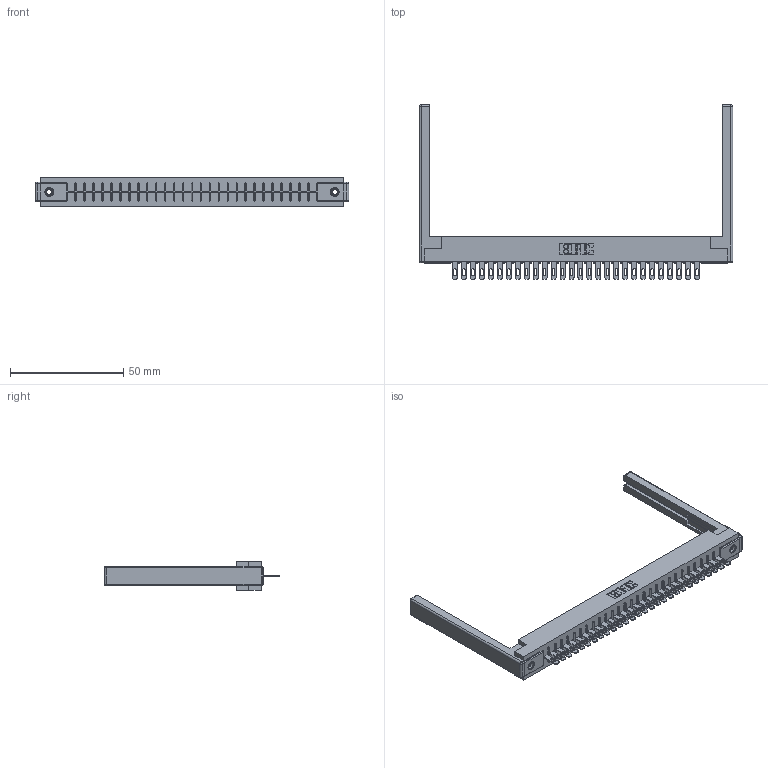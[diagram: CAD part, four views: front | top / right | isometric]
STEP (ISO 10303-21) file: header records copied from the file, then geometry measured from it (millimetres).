
FILE_DESCRIPTION (( 'STEP AP203' ), '1' );
FILE_NAME ('356-028-500-168.STEP', '2018-08-01T20:38:24', ( '' ), ( '' ), 'SwSTEP 2.0', 'SolidWorks 2016', '' );
FILE_SCHEMA (( 'CONFIG_CONTROL_DESIGN' ));
Length unit declared in the file: inch
Products named in the file (5): 306 Part_.156 Dia; 306-290-001_100; 345-250-001_345-250-001-102; 307-220-068; 356-028-500-168
Assembly tree (33 placements, depth 2):
  356-028-500-168
    306 Part_.156 Dia
    306-290-001_100  x28
    345-250-001_345-250-001-102  x2
    307-220-068  x2
Bounding box: 138.38 x 77.17 x 12.7 mm (x, y, z)
Volume: 19623.9 mm3; surface area: 20070.8 mm2
Topology: 33 solids, 33 shells, 2398 faces, 6726 edges, 4312 vertices
Faces by surface type: plane 1556, cylinder 706, sphere 120, cone 12, torus 4
Entity records: 30848 total; most frequent: CARTESIAN_POINT 5144, ORIENTED_EDGE 5090, DIRECTION 5087, EDGE_CURVE 2545, LINE 1977, VECTOR 1977, VERTEX_POINT 1612, AXIS2_PLACEMENT_3D 1555
